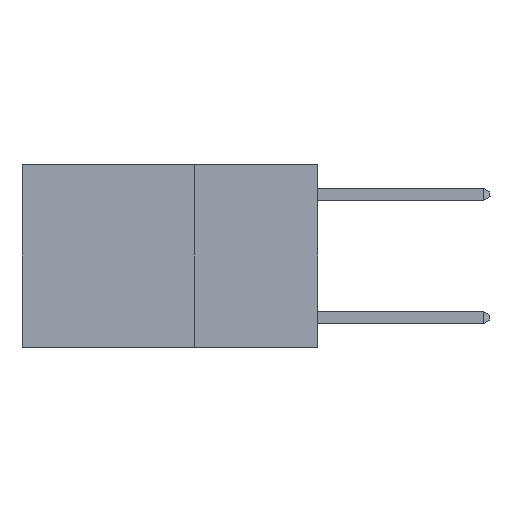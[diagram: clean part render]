
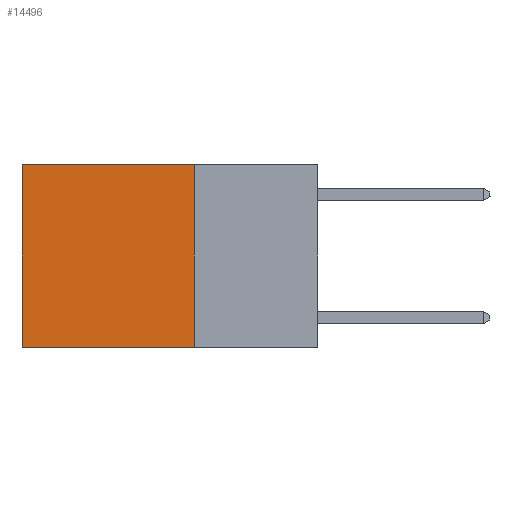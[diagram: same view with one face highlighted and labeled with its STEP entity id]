
A CAD part, left-side view. The second image highlights one B-rep face of the part: STEP entity #14496.
In plain terms, the highlighted planar face has unit normal (-1, 0, 0).
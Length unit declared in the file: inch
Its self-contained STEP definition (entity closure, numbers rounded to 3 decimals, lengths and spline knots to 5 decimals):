
#720 = VECTOR ( 'NONE', #12443, 39.37008 ) ;
#829 = CARTESIAN_POINT ( 'NONE',  ( 0.2625, 0.6, -0.37 ) ) ;
#925 = DIRECTION ( 'NONE',  ( 0., 1., 0. ) ) ;
#1199 = ORIENTED_EDGE ( 'NONE', *, *, #4607, .T. ) ;
#2356 = ORIENTED_EDGE ( 'NONE', *, *, #14370, .F. ) ;
#2703 = CARTESIAN_POINT ( 'NONE',  ( 0.2625, 0.25, -0.37 ) ) ;
#3322 = LINE ( 'NONE', #23770, #17637 ) ;
#3792 = LINE ( 'NONE', #3908, #6480 ) ;
#3839 = CARTESIAN_POINT ( 'NONE',  ( 0.2625, 0.25, 0. ) ) ;
#3908 = CARTESIAN_POINT ( 'NONE',  ( 0.2625, 0.25, 0. ) ) ;
#4106 = EDGE_CURVE ( 'NONE', #21218, #15535, #3322, .T. ) ;
#4607 = EDGE_CURVE ( 'NONE', #19618, #21218, #16046, .T. ) ;
#5478 = DIRECTION ( 'NONE',  ( 0., 0., -1. ) ) ;
#5721 = CARTESIAN_POINT ( 'NONE',  ( 0.2625, 0.25, 0. ) ) ;
#5728 = AXIS2_PLACEMENT_3D ( 'NONE', #3839, #9221, #5478 ) ;
#6480 = VECTOR ( 'NONE', #19135, 39.37008 ) ;
#8912 = EDGE_LOOP ( 'NONE', ( #21836, #23218, #2356, #1199 ) ) ;
#8975 = DIRECTION ( 'NONE',  ( 0., 0., -1. ) ) ;
#9221 = DIRECTION ( 'NONE',  ( 1., 0., 0. ) ) ;
#9346 = FACE_OUTER_BOUND ( 'NONE', #8912, .T. ) ;
#11717 = VECTOR ( 'NONE', #925, 39.37008 ) ;
#12100 = CARTESIAN_POINT ( 'NONE',  ( 0.2625, 0.6, 0. ) ) ;
#12443 = DIRECTION ( 'NONE',  ( 0., 1., 0. ) ) ;
#14370 = EDGE_CURVE ( 'NONE', #19618, #23117, #3792, .T. ) ;
#14496 = ADVANCED_FACE ( 'NONE', ( #9346 ), #15193, .F. ) ;
#15193 = PLANE ( 'NONE',  #5728 ) ;
#15535 = VERTEX_POINT ( 'NONE', #829 ) ;
#16046 = LINE ( 'NONE', #16542, #11717 ) ;
#16128 = EDGE_CURVE ( 'NONE', #23117, #15535, #18668, .T. ) ;
#16542 = CARTESIAN_POINT ( 'NONE',  ( 0.2625, 0.25, 0. ) ) ;
#17637 = VECTOR ( 'NONE', #8975, 39.37008 ) ;
#18668 = LINE ( 'NONE', #24255, #720 ) ;
#19135 = DIRECTION ( 'NONE',  ( 0., 0., -1. ) ) ;
#19618 = VERTEX_POINT ( 'NONE', #5721 ) ;
#21218 = VERTEX_POINT ( 'NONE', #12100 ) ;
#21836 = ORIENTED_EDGE ( 'NONE', *, *, #4106, .T. ) ;
#23117 = VERTEX_POINT ( 'NONE', #2703 ) ;
#23218 = ORIENTED_EDGE ( 'NONE', *, *, #16128, .F. ) ;
#23770 = CARTESIAN_POINT ( 'NONE',  ( 0.2625, 0.6, 0. ) ) ;
#24255 = CARTESIAN_POINT ( 'NONE',  ( 0.2625, 0.25, -0.37 ) ) ;
